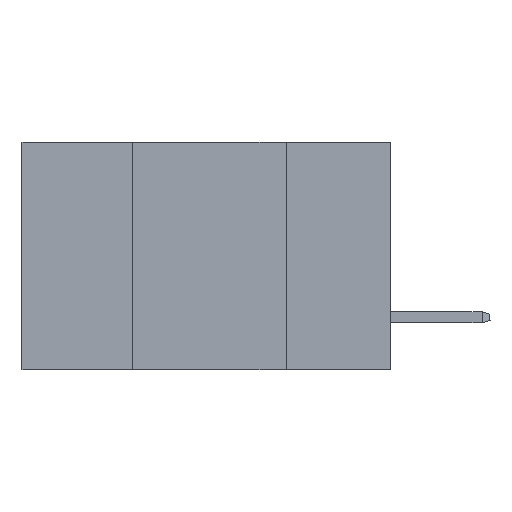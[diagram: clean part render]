
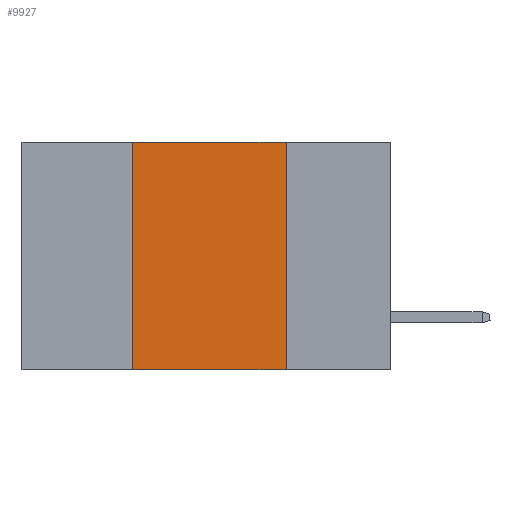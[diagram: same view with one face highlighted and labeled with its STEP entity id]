
A CAD part, left-side view. The second image highlights one B-rep face of the part: STEP entity #9927.
In plain terms, the highlighted planar face has unit normal (-1, 0, 0).
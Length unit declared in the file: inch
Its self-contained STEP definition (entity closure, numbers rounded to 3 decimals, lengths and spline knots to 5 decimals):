
#295 = ORIENTED_EDGE ( 'NONE', *, *, #7103, .T. ) ;
#741 = VERTEX_POINT ( 'NONE', #2322 ) ;
#867 = VERTEX_POINT ( 'NONE', #3915 ) ;
#1831 = LINE ( 'NONE', #10344, #6636 ) ;
#2322 = CARTESIAN_POINT ( 'NONE',  ( 0., 0.42, -0.37 ) ) ;
#2419 = FACE_OUTER_BOUND ( 'NONE', #7496, .T. ) ;
#2555 = DIRECTION ( 'NONE',  ( 0., -1., 0. ) ) ;
#3684 = EDGE_CURVE ( 'NONE', #741, #867, #1831, .T. ) ;
#3915 = CARTESIAN_POINT ( 'NONE',  ( 0., 0.42, 0. ) ) ;
#4020 = VECTOR ( 'NONE', #11418, 39.37008 ) ;
#4424 = ORIENTED_EDGE ( 'NONE', *, *, #3684, .F. ) ;
#4428 = CARTESIAN_POINT ( 'NONE',  ( 0., 0.6, 0. ) ) ;
#4681 = EDGE_CURVE ( 'NONE', #867, #6602, #6596, .T. ) ;
#5069 = DIRECTION ( 'NONE',  ( 0., 0., 1. ) ) ;
#5516 = VERTEX_POINT ( 'NONE', #8147 ) ;
#5891 = EDGE_CURVE ( 'NONE', #6602, #5516, #6174, .T. ) ;
#5900 = ORIENTED_EDGE ( 'NONE', *, *, #4681, .F. ) ;
#6013 = DIRECTION ( 'NONE',  ( 0., 0., -1. ) ) ;
#6137 = CARTESIAN_POINT ( 'NONE',  ( 0., 0.6, 0. ) ) ;
#6174 = LINE ( 'NONE', #11444, #4020 ) ;
#6411 = LINE ( 'NONE', #10504, #9910 ) ;
#6596 = LINE ( 'NONE', #6137, #10914 ) ;
#6602 = VERTEX_POINT ( 'NONE', #10634 ) ;
#6636 = VECTOR ( 'NONE', #5069, 39.37008 ) ;
#7103 = EDGE_CURVE ( 'NONE', #741, #5516, #6411, .T. ) ;
#7301 = ORIENTED_EDGE ( 'NONE', *, *, #5891, .F. ) ;
#7496 = EDGE_LOOP ( 'NONE', ( #7301, #5900, #4424, #295 ) ) ;
#8147 = CARTESIAN_POINT ( 'NONE',  ( 0., 0.17, -0.37 ) ) ;
#8469 = DIRECTION ( 'NONE',  ( 1., 0., 0. ) ) ;
#9910 = VECTOR ( 'NONE', #10662, 39.37008 ) ;
#9927 = ADVANCED_FACE ( 'NONE', ( #2419 ), #11355, .F. ) ;
#10344 = CARTESIAN_POINT ( 'NONE',  ( 0., 0.42, 0. ) ) ;
#10504 = CARTESIAN_POINT ( 'NONE',  ( 0., 0.6, -0.37 ) ) ;
#10634 = CARTESIAN_POINT ( 'NONE',  ( 0., 0.17, 0. ) ) ;
#10662 = DIRECTION ( 'NONE',  ( 0., -1., 0. ) ) ;
#10663 = AXIS2_PLACEMENT_3D ( 'NONE', #4428, #8469, #6013 ) ;
#10914 = VECTOR ( 'NONE', #2555, 39.37008 ) ;
#11355 = PLANE ( 'NONE',  #10663 ) ;
#11418 = DIRECTION ( 'NONE',  ( 0., 0., -1. ) ) ;
#11444 = CARTESIAN_POINT ( 'NONE',  ( 0., 0.17, 0. ) ) ;
